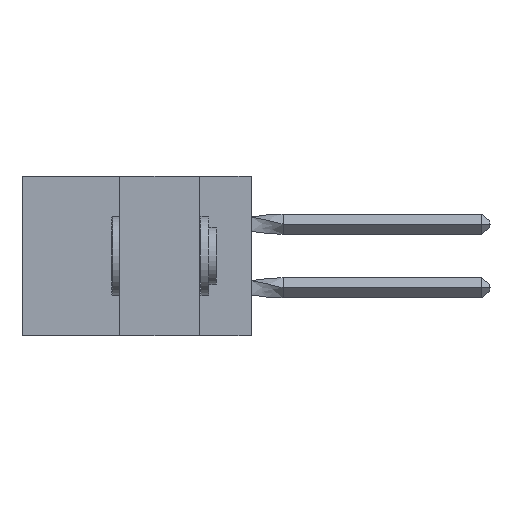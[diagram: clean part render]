
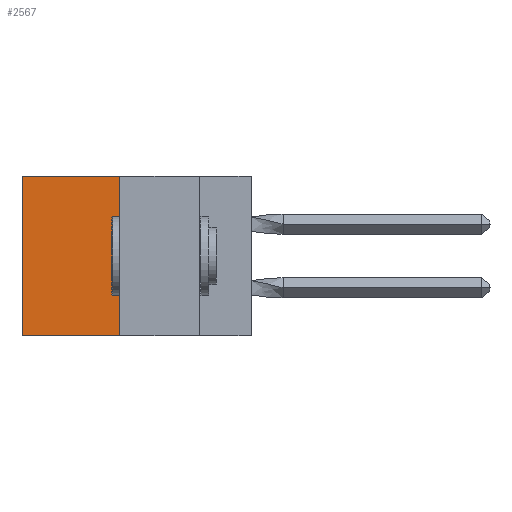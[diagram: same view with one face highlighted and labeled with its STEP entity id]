
A CAD part, left-side view. The second image highlights one B-rep face of the part: STEP entity #2567.
In plain terms, the highlighted planar face has unit normal (-1, 0, 0).
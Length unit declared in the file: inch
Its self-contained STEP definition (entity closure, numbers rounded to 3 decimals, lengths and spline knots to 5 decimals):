
#562 = VERTEX_POINT ( 'NONE', #10313 ) ;
#930 = VECTOR ( 'NONE', #18049, 39.37008 ) ;
#1039 = CARTESIAN_POINT ( 'NONE',  ( 0.305, 0.413, -0.5 ) ) ;
#2567 = ADVANCED_FACE ( 'NONE', ( #21483 ), #21222, .F. ) ;
#2647 = ORIENTED_EDGE ( 'NONE', *, *, #11053, .F. ) ;
#3692 = EDGE_LOOP ( 'NONE', ( #4263, #2647, #22804, #24142 ) ) ;
#3733 = VECTOR ( 'NONE', #16542, 39.37008 ) ;
#4263 = ORIENTED_EDGE ( 'NONE', *, *, #19246, .T. ) ;
#5048 = DIRECTION ( 'NONE',  ( 0., 0., -1. ) ) ;
#6229 = VERTEX_POINT ( 'NONE', #1039 ) ;
#6998 = CARTESIAN_POINT ( 'NONE',  ( 0.305, 0.413, 0. ) ) ;
#7661 = CARTESIAN_POINT ( 'NONE',  ( 0.305, 0.72, -0.5 ) ) ;
#8005 = CARTESIAN_POINT ( 'NONE',  ( 0.305, 0.72, 0. ) ) ;
#8361 = VECTOR ( 'NONE', #22967, 39.37008 ) ;
#8846 = LINE ( 'NONE', #6998, #3733 ) ;
#9760 = DIRECTION ( 'NONE',  ( 1., 0., 0. ) ) ;
#10313 = CARTESIAN_POINT ( 'NONE',  ( 0.305, 0.72, -0.5 ) ) ;
#11053 = EDGE_CURVE ( 'NONE', #6229, #562, #17383, .T. ) ;
#11637 = DIRECTION ( 'NONE',  ( 0., 0., -1. ) ) ;
#13170 = EDGE_CURVE ( 'NONE', #24804, #6229, #22625, .T. ) ;
#13544 = CARTESIAN_POINT ( 'NONE',  ( 0.305, 0.413, -0.5 ) ) ;
#15777 = CARTESIAN_POINT ( 'NONE',  ( 0.305, 0.413, 0. ) ) ;
#16331 = AXIS2_PLACEMENT_3D ( 'NONE', #13544, #9760, #11637 ) ;
#16542 = DIRECTION ( 'NONE',  ( 0., 1., 0. ) ) ;
#17383 = LINE ( 'NONE', #19870, #930 ) ;
#18049 = DIRECTION ( 'NONE',  ( 0., 1., 0. ) ) ;
#19246 = EDGE_CURVE ( 'NONE', #20738, #562, #24774, .T. ) ;
#19870 = CARTESIAN_POINT ( 'NONE',  ( 0.305, 0.413, -0.5 ) ) ;
#20738 = VERTEX_POINT ( 'NONE', #8005 ) ;
#21222 = PLANE ( 'NONE',  #16331 ) ;
#21483 = FACE_OUTER_BOUND ( 'NONE', #3692, .T. ) ;
#21742 = VECTOR ( 'NONE', #5048, 39.37008 ) ;
#22561 = EDGE_CURVE ( 'NONE', #24804, #20738, #8846, .T. ) ;
#22625 = LINE ( 'NONE', #23994, #21742 ) ;
#22804 = ORIENTED_EDGE ( 'NONE', *, *, #13170, .F. ) ;
#22967 = DIRECTION ( 'NONE',  ( 0., 0., -1. ) ) ;
#23994 = CARTESIAN_POINT ( 'NONE',  ( 0.305, 0.413, -0.5 ) ) ;
#24142 = ORIENTED_EDGE ( 'NONE', *, *, #22561, .T. ) ;
#24774 = LINE ( 'NONE', #7661, #8361 ) ;
#24804 = VERTEX_POINT ( 'NONE', #15777 ) ;
